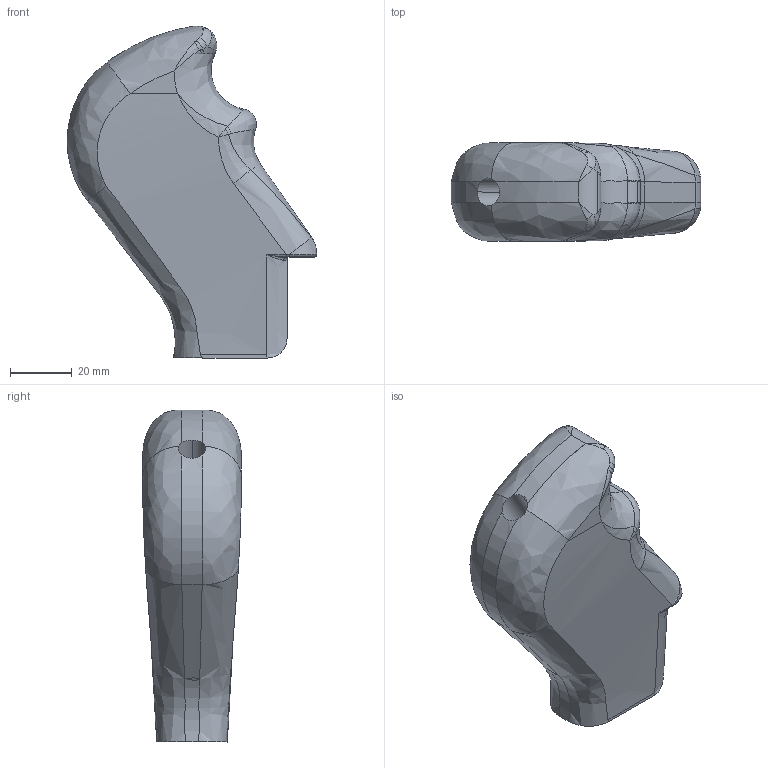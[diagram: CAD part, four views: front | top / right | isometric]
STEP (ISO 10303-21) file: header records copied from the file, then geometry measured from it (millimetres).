
FILE_DESCRIPTION (( 'STEP AP214' ), '1' );
FILE_NAME ('ThompsAR_Grip.step', '2015-04-02T12:14:45', ( 'WarFairy' ), ( '' ), 'SwSTEP 2.0', 'SolidWorks 2013', '' );
FILE_SCHEMA (( 'AUTOMOTIVE_DESIGN' ));
Length unit declared in the file: millimetre
Products named in the file (1): ThompsAR_Grip
Bounding box: 80.99 x 32 x 107.65 mm (x, y, z)
Volume: 127468.6 mm3; surface area: 20346 mm2
Topology: 1 solids, 1 shells, 109 faces, 307 edges, 193 vertices
Faces by surface type: bspline 64, cylinder 23, plane 22
Entity records: 8095 total; most frequent: CARTESIAN_POINT 5886, ORIENTED_EDGE 598, EDGE_CURVE 299, DIRECTION 252, VERTEX_POINT 193, B_SPLINE_CURVE_WITH_KNOTS 187, EDGE_LOOP 112, FACE_OUTER_BOUND 109
